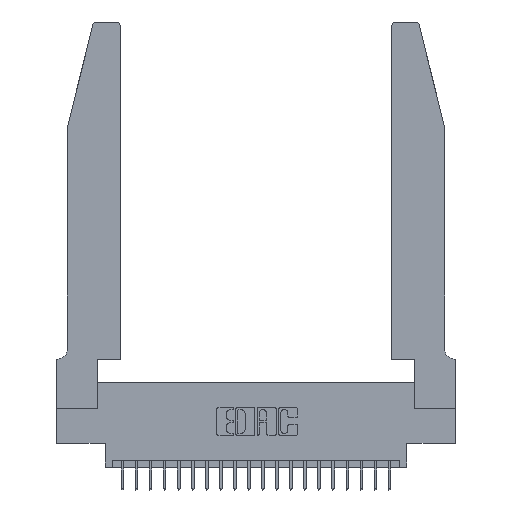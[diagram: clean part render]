
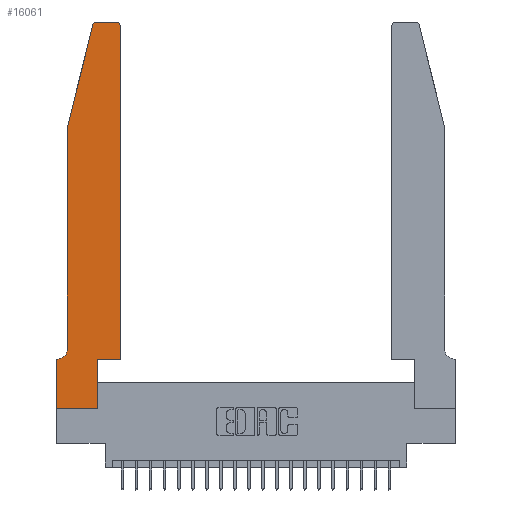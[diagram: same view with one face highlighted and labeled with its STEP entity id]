
A CAD part, top view. The second image highlights one B-rep face of the part: STEP entity #16061.
In plain terms, the highlighted planar face has unit normal (0, 0, 1).
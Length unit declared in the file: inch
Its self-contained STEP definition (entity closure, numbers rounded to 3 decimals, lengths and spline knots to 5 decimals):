
#231 = ORIENTED_EDGE ( 'NONE', *, *, #19572, .T. ) ;
#678 = CARTESIAN_POINT ( 'NONE',  ( 0.4505, 0.35, 0.37 ) ) ;
#1751 = CARTESIAN_POINT ( 'NONE',  ( 0.4205, 2.75, 0.37 ) ) ;
#1815 = CARTESIAN_POINT ( 'NONE',  ( 0.0755, 0.42, 0.37 ) ) ;
#1899 = AXIS2_PLACEMENT_3D ( 'NONE', #4876, #17578, #6728 ) ;
#1926 = DIRECTION ( 'NONE',  ( 0., 0., 1. ) ) ;
#2033 = CARTESIAN_POINT ( 'NONE',  ( 0.2865, 0.35, 0.37 ) ) ;
#2153 = CARTESIAN_POINT ( 'NONE',  ( 0.25487, 2.72718, 0.37 ) ) ;
#2166 = VERTEX_POINT ( 'NONE', #1815 ) ;
#2334 = ORIENTED_EDGE ( 'NONE', *, *, #15954, .T. ) ;
#3315 = VERTEX_POINT ( 'NONE', #1751 ) ;
#3957 = CARTESIAN_POINT ( 'NONE',  ( 0.4505, 2.72, 0.37 ) ) ;
#4031 = ORIENTED_EDGE ( 'NONE', *, *, #22694, .T. ) ;
#4630 = ORIENTED_EDGE ( 'NONE', *, *, #7960, .T. ) ;
#4698 = VECTOR ( 'NONE', #16041, 39.37008 ) ;
#4876 = CARTESIAN_POINT ( 'NONE',  ( 0., 0.35, 0.37 ) ) ;
#5431 = EDGE_CURVE ( 'NONE', #3315, #12209, #12265, .T. ) ;
#5643 = VERTEX_POINT ( 'NONE', #6829 ) ;
#5781 = EDGE_CURVE ( 'NONE', #8741, #7858, #10283, .T. ) ;
#5843 = DIRECTION ( 'NONE',  ( 0., 0., 1. ) ) ;
#6398 = LINE ( 'NONE', #7754, #20808 ) ;
#6630 = CARTESIAN_POINT ( 'NONE',  ( 0., 0.35, 0.37 ) ) ;
#6728 = DIRECTION ( 'NONE',  ( 1., 0., 0. ) ) ;
#6829 = CARTESIAN_POINT ( 'NONE',  ( 0.0755, 2., 0.37 ) ) ;
#6983 = ORIENTED_EDGE ( 'NONE', *, *, #16450, .T. ) ;
#7140 = CARTESIAN_POINT ( 'NONE',  ( 0., 0., 0.37 ) ) ;
#7299 = DIRECTION ( 'NONE',  ( 0., 1., 0. ) ) ;
#7629 = VERTEX_POINT ( 'NONE', #11986 ) ;
#7688 = VECTOR ( 'NONE', #20753, 39.37008 ) ;
#7754 = CARTESIAN_POINT ( 'NONE',  ( 0., 0., 0.37 ) ) ;
#7811 = CARTESIAN_POINT ( 'NONE',  ( 0., 0., 0.37 ) ) ;
#7812 = DIRECTION ( 'NONE',  ( -1., 0., 0. ) ) ;
#7854 = EDGE_CURVE ( 'NONE', #22792, #14211, #22915, .T. ) ;
#7858 = VERTEX_POINT ( 'NONE', #23399 ) ;
#7960 = EDGE_CURVE ( 'NONE', #18152, #3315, #10566, .T. ) ;
#8014 = DIRECTION ( 'NONE',  ( 0., 0., -1. ) ) ;
#8165 = AXIS2_PLACEMENT_3D ( 'NONE', #18850, #8014, #20612 ) ;
#8208 = AXIS2_PLACEMENT_3D ( 'NONE', #12996, #1926, #14828 ) ;
#8741 = VERTEX_POINT ( 'NONE', #7811 ) ;
#8829 = LINE ( 'NONE', #678, #7688 ) ;
#8955 = DIRECTION ( 'NONE',  ( -1., 0., 0. ) ) ;
#8979 = DIRECTION ( 'NONE',  ( 1., 0., 0. ) ) ;
#8996 = FACE_OUTER_BOUND ( 'NONE', #23039, .T. ) ;
#9049 = LINE ( 'NONE', #13738, #22827 ) ;
#9372 = CARTESIAN_POINT ( 'NONE',  ( 0.0055, 0.35, 0.37 ) ) ;
#9740 = EDGE_CURVE ( 'NONE', #12209, #17117, #17276, .T. ) ;
#10283 = LINE ( 'NONE', #7140, #19303 ) ;
#10371 = EDGE_CURVE ( 'NONE', #17117, #5643, #9049, .T. ) ;
#10566 = CIRCLE ( 'NONE', #8208, 0.03 ) ;
#11257 = EDGE_CURVE ( 'NONE', #7858, #19492, #14403, .T. ) ;
#11276 = LINE ( 'NONE', #22552, #16074 ) ;
#11384 = ORIENTED_EDGE ( 'NONE', *, *, #10371, .T. ) ;
#11461 = CARTESIAN_POINT ( 'NONE',  ( 0.2605, 2.75, 0.37 ) ) ;
#11676 = ORIENTED_EDGE ( 'NONE', *, *, #11257, .T. ) ;
#11830 = DIRECTION ( 'NONE',  ( 0., -1., 0. ) ) ;
#11986 = CARTESIAN_POINT ( 'NONE',  ( 0.4505, 0.35, 0.37 ) ) ;
#12025 = ORIENTED_EDGE ( 'NONE', *, *, #12854, .T. ) ;
#12082 = ORIENTED_EDGE ( 'NONE', *, *, #9740, .T. ) ;
#12209 = VERTEX_POINT ( 'NONE', #13744 ) ;
#12265 = LINE ( 'NONE', #11461, #20683 ) ;
#12854 = EDGE_CURVE ( 'NONE', #19492, #7629, #8829, .T. ) ;
#12996 = CARTESIAN_POINT ( 'NONE',  ( 0.4205, 2.72, 0.37 ) ) ;
#13738 = CARTESIAN_POINT ( 'NONE',  ( 0.0755, 2., 0.37 ) ) ;
#13744 = CARTESIAN_POINT ( 'NONE',  ( 0.284, 2.75, 0.37 ) ) ;
#14211 = VERTEX_POINT ( 'NONE', #6630 ) ;
#14403 = LINE ( 'NONE', #19582, #4698 ) ;
#14466 = AXIS2_PLACEMENT_3D ( 'NONE', #16701, #5843, #18509 ) ;
#14828 = DIRECTION ( 'NONE',  ( 1., 0., 0. ) ) ;
#14911 = CIRCLE ( 'NONE', #8165, 0.07 ) ;
#15541 = DIRECTION ( 'NONE',  ( -0.239, -0.971, 0. ) ) ;
#15954 = EDGE_CURVE ( 'NONE', #5643, #2166, #11276, .T. ) ;
#16041 = DIRECTION ( 'NONE',  ( 0., 1., 0. ) ) ;
#16061 = ADVANCED_FACE ( 'NONE', ( #8996 ), #21018, .T. ) ;
#16074 = VECTOR ( 'NONE', #11830, 39.37008 ) ;
#16450 = EDGE_CURVE ( 'NONE', #14211, #8741, #6398, .T. ) ;
#16498 = VECTOR ( 'NONE', #8955, 39.37008 ) ;
#16701 = CARTESIAN_POINT ( 'NONE',  ( 0.284, 2.72, 0.37 ) ) ;
#17117 = VERTEX_POINT ( 'NONE', #2153 ) ;
#17276 = CIRCLE ( 'NONE', #14466, 0.03 ) ;
#17578 = DIRECTION ( 'NONE',  ( 0., 0., 1. ) ) ;
#17803 = ORIENTED_EDGE ( 'NONE', *, *, #7854, .T. ) ;
#18028 = CARTESIAN_POINT ( 'NONE',  ( 0.0755, 0.35, 0.37 ) ) ;
#18128 = CARTESIAN_POINT ( 'NONE',  ( 0.4505, 0.35, 0.37 ) ) ;
#18152 = VERTEX_POINT ( 'NONE', #3957 ) ;
#18509 = DIRECTION ( 'NONE',  ( 1., 0., 0. ) ) ;
#18850 = CARTESIAN_POINT ( 'NONE',  ( 0.0055, 0.42, 0.37 ) ) ;
#19303 = VECTOR ( 'NONE', #8979, 39.37008 ) ;
#19492 = VERTEX_POINT ( 'NONE', #2033 ) ;
#19572 = EDGE_CURVE ( 'NONE', #2166, #22792, #14911, .T. ) ;
#19582 = CARTESIAN_POINT ( 'NONE',  ( 0.2865, 0.35, 0.37 ) ) ;
#20367 = DIRECTION ( 'NONE',  ( 0., -1., 0. ) ) ;
#20592 = ORIENTED_EDGE ( 'NONE', *, *, #5431, .T. ) ;
#20612 = DIRECTION ( 'NONE',  ( -1., 0., 0. ) ) ;
#20683 = VECTOR ( 'NONE', #7812, 39.37008 ) ;
#20753 = DIRECTION ( 'NONE',  ( 1., 0., 0. ) ) ;
#20808 = VECTOR ( 'NONE', #20367, 39.37008 ) ;
#21018 = PLANE ( 'NONE',  #1899 ) ;
#22060 = LINE ( 'NONE', #18128, #22613 ) ;
#22552 = CARTESIAN_POINT ( 'NONE',  ( 0.0755, 2., 0.37 ) ) ;
#22613 = VECTOR ( 'NONE', #7299, 39.37008 ) ;
#22694 = EDGE_CURVE ( 'NONE', #7629, #18152, #22060, .T. ) ;
#22792 = VERTEX_POINT ( 'NONE', #9372 ) ;
#22827 = VECTOR ( 'NONE', #15541, 39.37008 ) ;
#22915 = LINE ( 'NONE', #18028, #16498 ) ;
#23039 = EDGE_LOOP ( 'NONE', ( #20592, #12082, #11384, #2334, #231, #17803, #6983, #23455, #11676, #12025, #4031, #4630 ) ) ;
#23399 = CARTESIAN_POINT ( 'NONE',  ( 0.2865, 0., 0.37 ) ) ;
#23455 = ORIENTED_EDGE ( 'NONE', *, *, #5781, .T. ) ;
